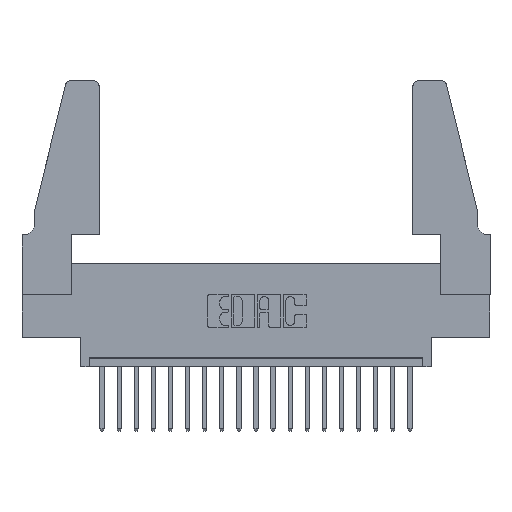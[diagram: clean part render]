
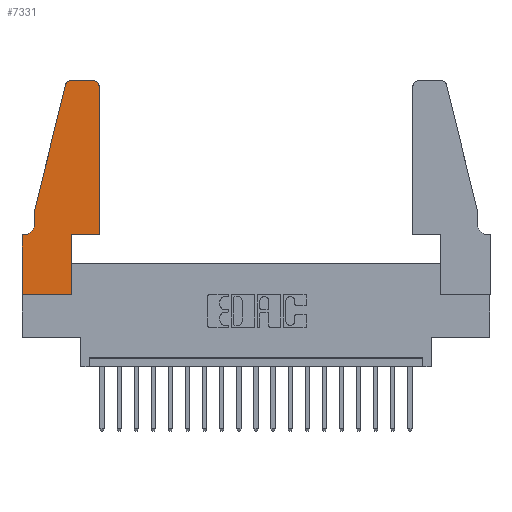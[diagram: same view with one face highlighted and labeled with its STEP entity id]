
A CAD part, top view. The second image highlights one B-rep face of the part: STEP entity #7331.
In plain terms, the highlighted planar face has unit normal (0, 0, 1).
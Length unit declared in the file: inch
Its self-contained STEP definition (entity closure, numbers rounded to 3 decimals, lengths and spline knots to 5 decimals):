
#29 = ORIENTED_EDGE ( 'NONE', *, *, #3331, .T. ) ;
#69 = PLANE ( 'NONE',  #17234 ) ;
#1033 = ORIENTED_EDGE ( 'NONE', *, *, #11530, .T. ) ;
#1059 = LINE ( 'NONE', #19588, #19392 ) ;
#1180 = VECTOR ( 'NONE', #12765, 39.37008 ) ;
#1433 = DIRECTION ( 'NONE',  ( 1., 0., 0. ) ) ;
#1922 = VERTEX_POINT ( 'NONE', #15442 ) ;
#2118 = CARTESIAN_POINT ( 'NONE',  ( 0.284, 1.25, 0.37 ) ) ;
#2660 = CARTESIAN_POINT ( 'NONE',  ( 0.4505, 0.35, 0.37 ) ) ;
#2965 = CARTESIAN_POINT ( 'NONE',  ( 0.2865, 0.35, 0.37 ) ) ;
#2969 = LINE ( 'NONE', #16816, #14156 ) ;
#2993 = CARTESIAN_POINT ( 'NONE',  ( 0., 0.35, 0.37 ) ) ;
#3258 = CARTESIAN_POINT ( 'NONE',  ( 0., 0.35, 0.37 ) ) ;
#3331 = EDGE_CURVE ( 'NONE', #13668, #8344, #8800, .T. ) ;
#3677 = VERTEX_POINT ( 'NONE', #19379 ) ;
#3869 = LINE ( 'NONE', #2965, #10808 ) ;
#3927 = CARTESIAN_POINT ( 'NONE',  ( 0.25487, 1.22718, 0.37 ) ) ;
#4016 = ORIENTED_EDGE ( 'NONE', *, *, #10101, .T. ) ;
#4048 = EDGE_CURVE ( 'NONE', #8344, #1922, #8120, .T. ) ;
#4148 = DIRECTION ( 'NONE',  ( 1., 0., 0. ) ) ;
#4484 = VERTEX_POINT ( 'NONE', #14070 ) ;
#4535 = DIRECTION ( 'NONE',  ( 0., 0., 1. ) ) ;
#4677 = DIRECTION ( 'NONE',  ( 1., 0., 0. ) ) ;
#5136 = VECTOR ( 'NONE', #4148, 39.37008 ) ;
#5161 = CARTESIAN_POINT ( 'NONE',  ( 0.0755, 0.42, 0.37 ) ) ;
#5798 = CARTESIAN_POINT ( 'NONE',  ( 0.4505, 0.35, 0.37 ) ) ;
#6326 = DIRECTION ( 'NONE',  ( 0., -1., 0. ) ) ;
#6370 = LINE ( 'NONE', #5798, #7333 ) ;
#6468 = ORIENTED_EDGE ( 'NONE', *, *, #8484, .T. ) ;
#6536 = ORIENTED_EDGE ( 'NONE', *, *, #9024, .T. ) ;
#6691 = ORIENTED_EDGE ( 'NONE', *, *, #8615, .T. ) ;
#6857 = DIRECTION ( 'NONE',  ( 0., -1., 0. ) ) ;
#6983 = CARTESIAN_POINT ( 'NONE',  ( 0.0755, 0.5, 0.37 ) ) ;
#7331 = ADVANCED_FACE ( 'NONE', ( #14465 ), #69, .T. ) ;
#7333 = VECTOR ( 'NONE', #10405, 39.37008 ) ;
#7549 = VERTEX_POINT ( 'NONE', #5161 ) ;
#7712 = DIRECTION ( 'NONE',  ( -1., 0., 0. ) ) ;
#8120 = LINE ( 'NONE', #15925, #10258 ) ;
#8248 = CARTESIAN_POINT ( 'NONE',  ( 0.0055, 0.35, 0.37 ) ) ;
#8344 = VERTEX_POINT ( 'NONE', #3258 ) ;
#8450 = VECTOR ( 'NONE', #18015, 39.37008 ) ;
#8484 = EDGE_CURVE ( 'NONE', #13537, #11180, #18674, .T. ) ;
#8615 = EDGE_CURVE ( 'NONE', #15135, #7549, #2969, .T. ) ;
#8800 = LINE ( 'NONE', #12693, #1180 ) ;
#9024 = EDGE_CURVE ( 'NONE', #9633, #3677, #3869, .T. ) ;
#9633 = VERTEX_POINT ( 'NONE', #17971 ) ;
#9721 = CARTESIAN_POINT ( 'NONE',  ( 0.0055, 0.42, 0.37 ) ) ;
#9783 = DIRECTION ( 'NONE',  ( -0.239, -0.971, 0. ) ) ;
#10101 = EDGE_CURVE ( 'NONE', #3677, #4484, #10148, .T. ) ;
#10148 = LINE ( 'NONE', #2660, #5136 ) ;
#10258 = VECTOR ( 'NONE', #6857, 39.37008 ) ;
#10288 = EDGE_CURVE ( 'NONE', #1922, #9633, #11093, .T. ) ;
#10343 = CARTESIAN_POINT ( 'NONE',  ( 0.284, 1.22, 0.37 ) ) ;
#10405 = DIRECTION ( 'NONE',  ( 0., 1., 0. ) ) ;
#10485 = CARTESIAN_POINT ( 'NONE',  ( 0., 0., 0.37 ) ) ;
#10512 = VERTEX_POINT ( 'NONE', #2118 ) ;
#10808 = VECTOR ( 'NONE', #13595, 39.37008 ) ;
#11093 = LINE ( 'NONE', #10485, #8450 ) ;
#11180 = VERTEX_POINT ( 'NONE', #12531 ) ;
#11530 = EDGE_CURVE ( 'NONE', #11180, #10512, #1059, .T. ) ;
#12023 = DIRECTION ( 'NONE',  ( 0., 0., 1. ) ) ;
#12034 = ORIENTED_EDGE ( 'NONE', *, *, #4048, .T. ) ;
#12304 = DIRECTION ( 'NONE',  ( 0., 0., 1. ) ) ;
#12531 = CARTESIAN_POINT ( 'NONE',  ( 0.4205, 1.25, 0.37 ) ) ;
#12693 = CARTESIAN_POINT ( 'NONE',  ( 0.0755, 0.35, 0.37 ) ) ;
#12765 = DIRECTION ( 'NONE',  ( -1., 0., 0. ) ) ;
#12822 = ORIENTED_EDGE ( 'NONE', *, *, #19084, .T. ) ;
#13153 = ORIENTED_EDGE ( 'NONE', *, *, #18100, .T. ) ;
#13237 = VECTOR ( 'NONE', #9783, 39.37008 ) ;
#13537 = VERTEX_POINT ( 'NONE', #17259 ) ;
#13595 = DIRECTION ( 'NONE',  ( 0., 1., 0. ) ) ;
#13668 = VERTEX_POINT ( 'NONE', #8248 ) ;
#13745 = CARTESIAN_POINT ( 'NONE',  ( 0.4205, 1.22, 0.37 ) ) ;
#13912 = CARTESIAN_POINT ( 'NONE',  ( 0.0755, 0.5, 0.37 ) ) ;
#13995 = AXIS2_PLACEMENT_3D ( 'NONE', #10343, #12023, #1433 ) ;
#14070 = CARTESIAN_POINT ( 'NONE',  ( 0.4505, 0.35, 0.37 ) ) ;
#14156 = VECTOR ( 'NONE', #6326, 39.37008 ) ;
#14166 = CIRCLE ( 'NONE', #16105, 0.07 ) ;
#14465 = FACE_OUTER_BOUND ( 'NONE', #18929, .T. ) ;
#15135 = VERTEX_POINT ( 'NONE', #6983 ) ;
#15442 = CARTESIAN_POINT ( 'NONE',  ( 0., 0., 0.37 ) ) ;
#15612 = EDGE_CURVE ( 'NONE', #7549, #13668, #14166, .T. ) ;
#15663 = ORIENTED_EDGE ( 'NONE', *, *, #15612, .T. ) ;
#15906 = DIRECTION ( 'NONE',  ( -1., 0., 0. ) ) ;
#15925 = CARTESIAN_POINT ( 'NONE',  ( 0., 0., 0.37 ) ) ;
#16033 = CIRCLE ( 'NONE', #13995, 0.03 ) ;
#16105 = AXIS2_PLACEMENT_3D ( 'NONE', #9721, #18916, #15906 ) ;
#16498 = EDGE_CURVE ( 'NONE', #4484, #13537, #6370, .T. ) ;
#16672 = AXIS2_PLACEMENT_3D ( 'NONE', #13745, #4535, #18077 ) ;
#16816 = CARTESIAN_POINT ( 'NONE',  ( 0.0755, 0.5, 0.37 ) ) ;
#17234 = AXIS2_PLACEMENT_3D ( 'NONE', #2993, #12304, #4677 ) ;
#17259 = CARTESIAN_POINT ( 'NONE',  ( 0.4505, 1.22, 0.37 ) ) ;
#17306 = LINE ( 'NONE', #13912, #13237 ) ;
#17971 = CARTESIAN_POINT ( 'NONE',  ( 0.2865, 0., 0.37 ) ) ;
#18015 = DIRECTION ( 'NONE',  ( 1., 0., 0. ) ) ;
#18077 = DIRECTION ( 'NONE',  ( 1., 0., 0. ) ) ;
#18100 = EDGE_CURVE ( 'NONE', #19531, #15135, #17306, .T. ) ;
#18580 = ORIENTED_EDGE ( 'NONE', *, *, #10288, .T. ) ;
#18601 = ORIENTED_EDGE ( 'NONE', *, *, #16498, .T. ) ;
#18674 = CIRCLE ( 'NONE', #16672, 0.03 ) ;
#18916 = DIRECTION ( 'NONE',  ( 0., 0., -1. ) ) ;
#18929 = EDGE_LOOP ( 'NONE', ( #1033, #12822, #13153, #6691, #15663, #29, #12034, #18580, #6536, #4016, #18601, #6468 ) ) ;
#19084 = EDGE_CURVE ( 'NONE', #10512, #19531, #16033, .T. ) ;
#19379 = CARTESIAN_POINT ( 'NONE',  ( 0.2865, 0.35, 0.37 ) ) ;
#19392 = VECTOR ( 'NONE', #7712, 39.37008 ) ;
#19531 = VERTEX_POINT ( 'NONE', #3927 ) ;
#19588 = CARTESIAN_POINT ( 'NONE',  ( 0.2605, 1.25, 0.37 ) ) ;
